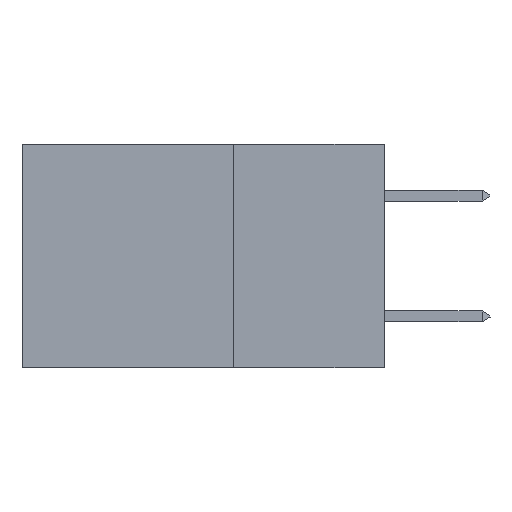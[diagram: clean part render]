
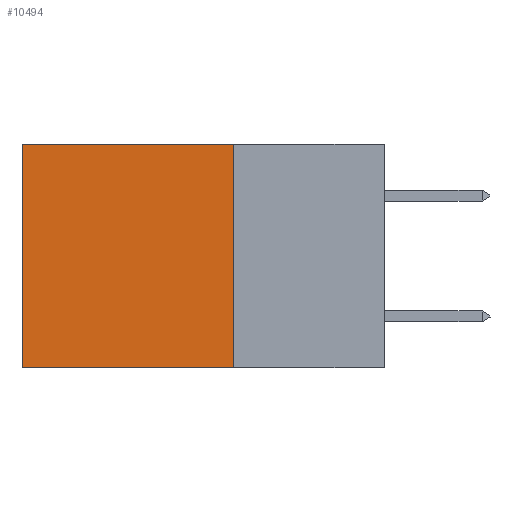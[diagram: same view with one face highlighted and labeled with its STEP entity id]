
A CAD part, left-side view. The second image highlights one B-rep face of the part: STEP entity #10494.
In plain terms, the highlighted planar face has unit normal (-1, 0, 0).
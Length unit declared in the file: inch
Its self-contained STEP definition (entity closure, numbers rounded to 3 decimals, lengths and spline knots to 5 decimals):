
#650 = DIRECTION ( 'NONE',  ( 1., 0., 0. ) ) ;
#807 = CARTESIAN_POINT ( 'NONE',  ( 0.2875, 0.25, -0.37 ) ) ;
#853 = VERTEX_POINT ( 'NONE', #8438 ) ;
#1565 = ORIENTED_EDGE ( 'NONE', *, *, #2283, .F. ) ;
#2283 = EDGE_CURVE ( 'NONE', #853, #10547, #9881, .T. ) ;
#3523 = EDGE_CURVE ( 'NONE', #9814, #15399, #5548, .T. ) ;
#3581 = VECTOR ( 'NONE', #15492, 39.37008 ) ;
#3862 = DIRECTION ( 'NONE',  ( 0., 0., -1. ) ) ;
#4444 = CARTESIAN_POINT ( 'NONE',  ( 0.2875, 0.6, 0. ) ) ;
#4497 = CARTESIAN_POINT ( 'NONE',  ( 0.2875, 0.6, -0.37 ) ) ;
#5539 = FACE_OUTER_BOUND ( 'NONE', #8534, .T. ) ;
#5548 = LINE ( 'NONE', #13346, #11533 ) ;
#5655 = EDGE_CURVE ( 'NONE', #853, #9814, #9042, .T. ) ;
#5950 = CARTESIAN_POINT ( 'NONE',  ( 0.2875, 0.25, 0. ) ) ;
#6510 = VECTOR ( 'NONE', #8635, 39.37008 ) ;
#7250 = ORIENTED_EDGE ( 'NONE', *, *, #5655, .T. ) ;
#8424 = ORIENTED_EDGE ( 'NONE', *, *, #11859, .F. ) ;
#8438 = CARTESIAN_POINT ( 'NONE',  ( 0.2875, 0.25, 0. ) ) ;
#8534 = EDGE_LOOP ( 'NONE', ( #14304, #8424, #1565, #7250 ) ) ;
#8635 = DIRECTION ( 'NONE',  ( 0., 1., 0. ) ) ;
#9042 = LINE ( 'NONE', #5950, #3581 ) ;
#9131 = DIRECTION ( 'NONE',  ( 0., 0., -1. ) ) ;
#9721 = DIRECTION ( 'NONE',  ( 0., 0., -1. ) ) ;
#9814 = VERTEX_POINT ( 'NONE', #4444 ) ;
#9881 = LINE ( 'NONE', #11089, #13060 ) ;
#10222 = CARTESIAN_POINT ( 'NONE',  ( 0.2875, 0.25, 0. ) ) ;
#10446 = LINE ( 'NONE', #13379, #6510 ) ;
#10494 = ADVANCED_FACE ( 'NONE', ( #5539 ), #14970, .F. ) ;
#10547 = VERTEX_POINT ( 'NONE', #807 ) ;
#11089 = CARTESIAN_POINT ( 'NONE',  ( 0.2875, 0.25, 0. ) ) ;
#11533 = VECTOR ( 'NONE', #9721, 39.37008 ) ;
#11859 = EDGE_CURVE ( 'NONE', #10547, #15399, #10446, .T. ) ;
#12982 = AXIS2_PLACEMENT_3D ( 'NONE', #10222, #650, #9131 ) ;
#13060 = VECTOR ( 'NONE', #3862, 39.37008 ) ;
#13346 = CARTESIAN_POINT ( 'NONE',  ( 0.2875, 0.6, 0. ) ) ;
#13379 = CARTESIAN_POINT ( 'NONE',  ( 0.2875, 0.25, -0.37 ) ) ;
#14304 = ORIENTED_EDGE ( 'NONE', *, *, #3523, .T. ) ;
#14970 = PLANE ( 'NONE',  #12982 ) ;
#15399 = VERTEX_POINT ( 'NONE', #4497 ) ;
#15492 = DIRECTION ( 'NONE',  ( 0., 1., 0. ) ) ;
